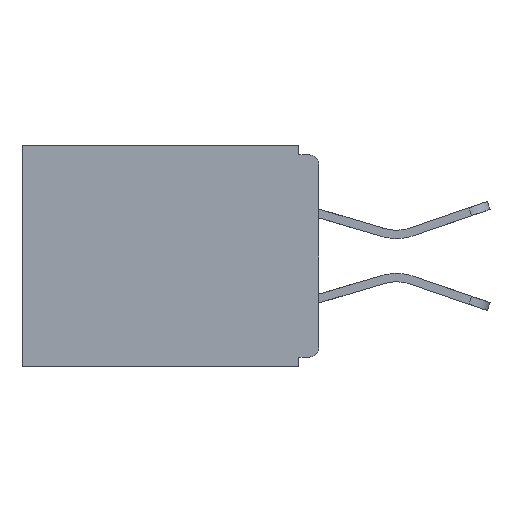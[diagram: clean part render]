
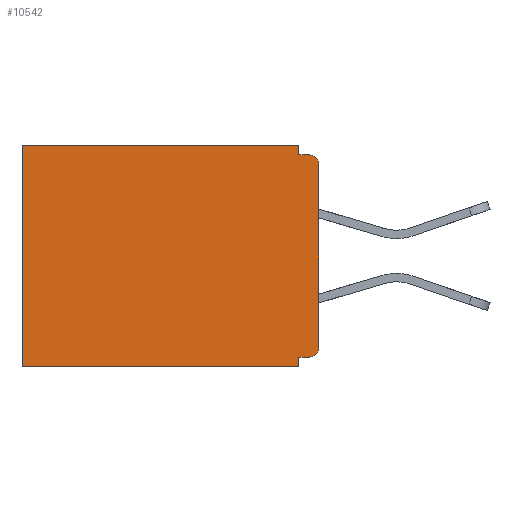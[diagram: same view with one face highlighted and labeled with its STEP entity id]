
A CAD part, left-side view. The second image highlights one B-rep face of the part: STEP entity #10542.
In plain terms, the highlighted planar face has unit normal (-1, 0, 0).
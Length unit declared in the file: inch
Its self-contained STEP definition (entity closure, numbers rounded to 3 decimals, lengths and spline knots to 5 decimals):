
#130 = CIRCLE ( 'NONE', #5932, 0.015 ) ;
#437 = EDGE_CURVE ( 'NONE', #18077, #3636, #12923, .T. ) ;
#745 = CARTESIAN_POINT ( 'NONE',  ( 0.298, 0.015, -0.328 ) ) ;
#990 = PLANE ( 'NONE',  #12935 ) ;
#1848 = DIRECTION ( 'NONE',  ( 0., 0., -1. ) ) ;
#1908 = DIRECTION ( 'NONE',  ( 0., 0., -1. ) ) ;
#2498 = EDGE_CURVE ( 'NONE', #13548, #4011, #18582, .T. ) ;
#2545 = VERTEX_POINT ( 'NONE', #3582 ) ;
#2630 = ORIENTED_EDGE ( 'NONE', *, *, #437, .F. ) ;
#2778 = CARTESIAN_POINT ( 'NONE',  ( 0.298, 0.031, 0. ) ) ;
#3073 = VECTOR ( 'NONE', #4342, 39.37008 ) ;
#3582 = CARTESIAN_POINT ( 'NONE',  ( 0.298, 0.031, -0.015 ) ) ;
#3636 = VERTEX_POINT ( 'NONE', #8685 ) ;
#3712 = EDGE_LOOP ( 'NONE', ( #6682, #16007, #15870, #13603, #13790, #16949, #4268, #2630, #7548, #5857 ) ) ;
#3739 = CARTESIAN_POINT ( 'NONE',  ( 0.298, 0.46, 0. ) ) ;
#4011 = VERTEX_POINT ( 'NONE', #15888 ) ;
#4268 = ORIENTED_EDGE ( 'NONE', *, *, #14828, .F. ) ;
#4342 = DIRECTION ( 'NONE',  ( 0., 1., 0. ) ) ;
#4559 = EDGE_CURVE ( 'NONE', #19191, #16975, #13424, .T. ) ;
#4740 = LINE ( 'NONE', #9563, #7875 ) ;
#5151 = CARTESIAN_POINT ( 'NONE',  ( 0.298, 0.46, -0.343 ) ) ;
#5640 = CARTESIAN_POINT ( 'NONE',  ( 0.298, 0., -0.343 ) ) ;
#5857 = ORIENTED_EDGE ( 'NONE', *, *, #2498, .F. ) ;
#5932 = AXIS2_PLACEMENT_3D ( 'NONE', #19613, #18238, #13730 ) ;
#6396 = CARTESIAN_POINT ( 'NONE',  ( 0.298, 0., -0.328 ) ) ;
#6399 = DIRECTION ( 'NONE',  ( -1., 0., 0. ) ) ;
#6437 = DIRECTION ( 'NONE',  ( 0., 0., -1. ) ) ;
#6523 = VERTEX_POINT ( 'NONE', #16682 ) ;
#6600 = EDGE_CURVE ( 'NONE', #13545, #19191, #4740, .T. ) ;
#6682 = ORIENTED_EDGE ( 'NONE', *, *, #8814, .T. ) ;
#6743 = VERTEX_POINT ( 'NONE', #13695 ) ;
#7444 = VECTOR ( 'NONE', #19005, 39.37008 ) ;
#7548 = ORIENTED_EDGE ( 'NONE', *, *, #19460, .T. ) ;
#7816 = VECTOR ( 'NONE', #1908, 39.37008 ) ;
#7875 = VECTOR ( 'NONE', #8404, 39.37008 ) ;
#8404 = DIRECTION ( 'NONE',  ( 0., 1., 0. ) ) ;
#8459 = DIRECTION ( 'NONE',  ( 1., 0., 0. ) ) ;
#8685 = CARTESIAN_POINT ( 'NONE',  ( 0.298, 0.031, -0.328 ) ) ;
#8814 = EDGE_CURVE ( 'NONE', #13548, #6523, #14948, .T. ) ;
#9048 = DIRECTION ( 'NONE',  ( 0., -1., 0. ) ) ;
#9563 = CARTESIAN_POINT ( 'NONE',  ( 0.298, 0., 0. ) ) ;
#9714 = VECTOR ( 'NONE', #9048, 39.37008 ) ;
#10002 = DIRECTION ( 'NONE',  ( 0., 0., -1. ) ) ;
#10542 = ADVANCED_FACE ( 'NONE', ( #14397 ), #990, .F. ) ;
#10908 = CARTESIAN_POINT ( 'NONE',  ( 0.298, 0.031, -0.343 ) ) ;
#12211 = CARTESIAN_POINT ( 'NONE',  ( 0.298, 0., -0.03 ) ) ;
#12268 = CARTESIAN_POINT ( 'NONE',  ( 0.298, 0., -0.015 ) ) ;
#12450 = VECTOR ( 'NONE', #18634, 39.37008 ) ;
#12923 = LINE ( 'NONE', #6396, #12450 ) ;
#12935 = AXIS2_PLACEMENT_3D ( 'NONE', #17829, #8459, #19051 ) ;
#12949 = CARTESIAN_POINT ( 'NONE',  ( 0.298, 0.031, -0.343 ) ) ;
#13424 = LINE ( 'NONE', #3739, #7444 ) ;
#13545 = VERTEX_POINT ( 'NONE', #2778 ) ;
#13548 = VERTEX_POINT ( 'NONE', #12211 ) ;
#13603 = ORIENTED_EDGE ( 'NONE', *, *, #6600, .T. ) ;
#13634 = EDGE_CURVE ( 'NONE', #6743, #16975, #18630, .T. ) ;
#13695 = CARTESIAN_POINT ( 'NONE',  ( 0.298, 0.031, -0.343 ) ) ;
#13730 = DIRECTION ( 'NONE',  ( 0., 0., -1. ) ) ;
#13790 = ORIENTED_EDGE ( 'NONE', *, *, #4559, .T. ) ;
#14397 = FACE_OUTER_BOUND ( 'NONE', #3712, .T. ) ;
#14534 = CARTESIAN_POINT ( 'NONE',  ( 0.298, 0.015, -0.03 ) ) ;
#14737 = LINE ( 'NONE', #12949, #15712 ) ;
#14746 = EDGE_CURVE ( 'NONE', #2545, #6523, #16433, .T. ) ;
#14828 = EDGE_CURVE ( 'NONE', #3636, #6743, #19561, .T. ) ;
#14948 = CIRCLE ( 'NONE', #18696, 0.015 ) ;
#15712 = VECTOR ( 'NONE', #10002, 39.37008 ) ;
#15870 = ORIENTED_EDGE ( 'NONE', *, *, #19495, .F. ) ;
#15888 = CARTESIAN_POINT ( 'NONE',  ( 0.298, 0., -0.313 ) ) ;
#16007 = ORIENTED_EDGE ( 'NONE', *, *, #14746, .F. ) ;
#16433 = LINE ( 'NONE', #12268, #9714 ) ;
#16682 = CARTESIAN_POINT ( 'NONE',  ( 0.298, 0.015, -0.015 ) ) ;
#16949 = ORIENTED_EDGE ( 'NONE', *, *, #13634, .F. ) ;
#16975 = VERTEX_POINT ( 'NONE', #5151 ) ;
#17168 = CARTESIAN_POINT ( 'NONE',  ( 0.298, 0., 0. ) ) ;
#17829 = CARTESIAN_POINT ( 'NONE',  ( 0.298, 0., 0. ) ) ;
#18077 = VERTEX_POINT ( 'NONE', #745 ) ;
#18092 = VECTOR ( 'NONE', #6437, 39.37008 ) ;
#18238 = DIRECTION ( 'NONE',  ( -1., 0., 0. ) ) ;
#18582 = LINE ( 'NONE', #17168, #7816 ) ;
#18630 = LINE ( 'NONE', #5640, #3073 ) ;
#18634 = DIRECTION ( 'NONE',  ( 0., 1., 0. ) ) ;
#18696 = AXIS2_PLACEMENT_3D ( 'NONE', #14534, #6399, #1848 ) ;
#19005 = DIRECTION ( 'NONE',  ( 0., 0., -1. ) ) ;
#19051 = DIRECTION ( 'NONE',  ( 0., 0., -1. ) ) ;
#19191 = VERTEX_POINT ( 'NONE', #19208 ) ;
#19208 = CARTESIAN_POINT ( 'NONE',  ( 0.298, 0.46, 0. ) ) ;
#19460 = EDGE_CURVE ( 'NONE', #18077, #4011, #130, .T. ) ;
#19495 = EDGE_CURVE ( 'NONE', #13545, #2545, #14737, .T. ) ;
#19561 = LINE ( 'NONE', #10908, #18092 ) ;
#19613 = CARTESIAN_POINT ( 'NONE',  ( 0.298, 0.015, -0.313 ) ) ;
